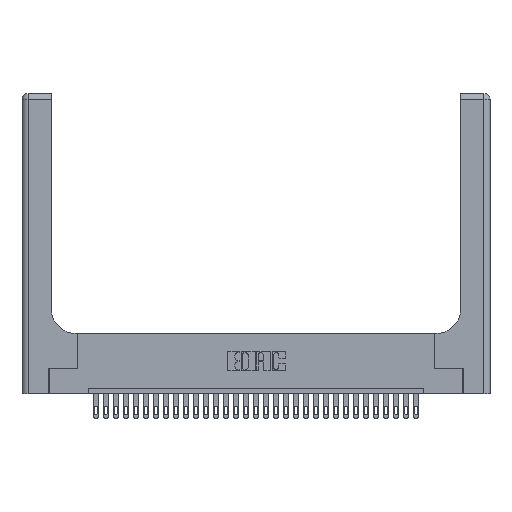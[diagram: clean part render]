
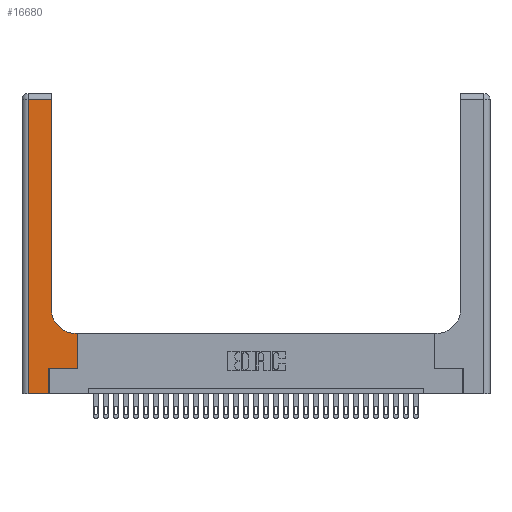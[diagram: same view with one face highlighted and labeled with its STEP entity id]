
A CAD part, top view. The second image highlights one B-rep face of the part: STEP entity #16680.
In plain terms, the highlighted planar face has unit normal (0, 0, 1).
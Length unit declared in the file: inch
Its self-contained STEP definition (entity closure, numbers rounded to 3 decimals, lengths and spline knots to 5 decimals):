
#653 = CARTESIAN_POINT ( 'NONE',  ( 0.2915, 3., 0.37 ) ) ;
#688 = VERTEX_POINT ( 'NONE', #6869 ) ;
#907 = DIRECTION ( 'NONE',  ( -1., 0., 0. ) ) ;
#1330 = ORIENTED_EDGE ( 'NONE', *, *, #17943, .T. ) ;
#1447 = CARTESIAN_POINT ( 'NONE',  ( 0.5415, 0.6, 0.37 ) ) ;
#1498 = DIRECTION ( 'NONE',  ( 0., 0., -1. ) ) ;
#3628 = CARTESIAN_POINT ( 'NONE',  ( 0.2915, 0.85, 0.37 ) ) ;
#3691 = LINE ( 'NONE', #653, #22106 ) ;
#4813 = PLANE ( 'NONE',  #30777 ) ;
#5582 = DIRECTION ( 'NONE',  ( 0., 1., 0. ) ) ;
#5802 = VECTOR ( 'NONE', #12513, 39.37008 ) ;
#6184 = VERTEX_POINT ( 'NONE', #26454 ) ;
#6189 = EDGE_CURVE ( 'NONE', #15887, #24402, #13624, .T. ) ;
#6240 = VECTOR ( 'NONE', #15672, 39.37008 ) ;
#6869 = CARTESIAN_POINT ( 'NONE',  ( 0.5585, 0.25, 0.37 ) ) ;
#6893 = CARTESIAN_POINT ( 'NONE',  ( 0., 0., 0.37 ) ) ;
#6897 = ORIENTED_EDGE ( 'NONE', *, *, #6189, .T. ) ;
#6902 = LINE ( 'NONE', #23848, #26499 ) ;
#6960 = DIRECTION ( 'NONE',  ( 1., 0., 0. ) ) ;
#7021 = AXIS2_PLACEMENT_3D ( 'NONE', #13616, #1498, #25425 ) ;
#7666 = DIRECTION ( 'NONE',  ( -1., 0., 0. ) ) ;
#7793 = VERTEX_POINT ( 'NONE', #1447 ) ;
#8768 = ORIENTED_EDGE ( 'NONE', *, *, #16784, .T. ) ;
#9126 = VECTOR ( 'NONE', #907, 39.37008 ) ;
#10651 = VECTOR ( 'NONE', #16989, 39.37008 ) ;
#10754 = EDGE_CURVE ( 'NONE', #24402, #30688, #6902, .T. ) ;
#11161 = EDGE_CURVE ( 'NONE', #7793, #23447, #12227, .T. ) ;
#11666 = LINE ( 'NONE', #14273, #12425 ) ;
#11920 = DIRECTION ( 'NONE',  ( 0., -1., 0. ) ) ;
#12227 = CIRCLE ( 'NONE', #7021, 0.25 ) ;
#12425 = VECTOR ( 'NONE', #6960, 39.37008 ) ;
#12513 = DIRECTION ( 'NONE',  ( 0., 1., 0. ) ) ;
#13601 = EDGE_LOOP ( 'NONE', ( #8768, #25723, #25449, #6897, #31144, #28677, #14193, #1330, #15732 ) ) ;
#13616 = CARTESIAN_POINT ( 'NONE',  ( 0.5415, 0.85, 0.37 ) ) ;
#13624 = LINE ( 'NONE', #6893, #10651 ) ;
#14193 = ORIENTED_EDGE ( 'NONE', *, *, #29906, .T. ) ;
#14273 = CARTESIAN_POINT ( 'NONE',  ( 0.269, 0.25, 0.37 ) ) ;
#14538 = EDGE_CURVE ( 'NONE', #21048, #15887, #25951, .T. ) ;
#15152 = CARTESIAN_POINT ( 'NONE',  ( 0.2915, 0.6, 0.37 ) ) ;
#15672 = DIRECTION ( 'NONE',  ( -1., 0., 0. ) ) ;
#15732 = ORIENTED_EDGE ( 'NONE', *, *, #11161, .T. ) ;
#15887 = VERTEX_POINT ( 'NONE', #17524 ) ;
#15949 = VERTEX_POINT ( 'NONE', #25364 ) ;
#16680 = ADVANCED_FACE ( 'NONE', ( #27053 ), #4813, .F. ) ;
#16784 = EDGE_CURVE ( 'NONE', #23447, #15949, #3691, .T. ) ;
#16989 = DIRECTION ( 'NONE',  ( 1., 0., 0. ) ) ;
#17524 = CARTESIAN_POINT ( 'NONE',  ( 0.06, 0., 0.37 ) ) ;
#17818 = LINE ( 'NONE', #24427, #5802 ) ;
#17943 = EDGE_CURVE ( 'NONE', #6184, #7793, #22686, .T. ) ;
#18243 = CARTESIAN_POINT ( 'NONE',  ( 0.269, 0.25, 0.37 ) ) ;
#19518 = EDGE_CURVE ( 'NONE', #30688, #688, #11666, .T. ) ;
#20526 = LINE ( 'NONE', #22747, #6240 ) ;
#21048 = VERTEX_POINT ( 'NONE', #30286 ) ;
#21851 = CARTESIAN_POINT ( 'NONE',  ( 0., 3., 0.37 ) ) ;
#22106 = VECTOR ( 'NONE', #5582, 39.37008 ) ;
#22244 = EDGE_CURVE ( 'NONE', #15949, #21048, #20526, .T. ) ;
#22686 = LINE ( 'NONE', #15152, #9126 ) ;
#22747 = CARTESIAN_POINT ( 'NONE',  ( 0., 2.94, 0.37 ) ) ;
#23447 = VERTEX_POINT ( 'NONE', #3628 ) ;
#23787 = DIRECTION ( 'NONE',  ( 0., 0., -1. ) ) ;
#23848 = CARTESIAN_POINT ( 'NONE',  ( 0.269, 0., 0.37 ) ) ;
#24402 = VERTEX_POINT ( 'NONE', #24681 ) ;
#24427 = CARTESIAN_POINT ( 'NONE',  ( 0.5585, 0.25, 0.37 ) ) ;
#24681 = CARTESIAN_POINT ( 'NONE',  ( 0.269, 0., 0.37 ) ) ;
#25364 = CARTESIAN_POINT ( 'NONE',  ( 0.2915, 2.94, 0.37 ) ) ;
#25425 = DIRECTION ( 'NONE',  ( 1., 0., 0. ) ) ;
#25449 = ORIENTED_EDGE ( 'NONE', *, *, #14538, .T. ) ;
#25723 = ORIENTED_EDGE ( 'NONE', *, *, #22244, .T. ) ;
#25951 = LINE ( 'NONE', #28609, #26745 ) ;
#26454 = CARTESIAN_POINT ( 'NONE',  ( 0.5585, 0.6, 0.37 ) ) ;
#26499 = VECTOR ( 'NONE', #28412, 39.37008 ) ;
#26745 = VECTOR ( 'NONE', #11920, 39.37008 ) ;
#27053 = FACE_OUTER_BOUND ( 'NONE', #13601, .T. ) ;
#28412 = DIRECTION ( 'NONE',  ( 0., 1., 0. ) ) ;
#28609 = CARTESIAN_POINT ( 'NONE',  ( 0.06, 3., 0.37 ) ) ;
#28677 = ORIENTED_EDGE ( 'NONE', *, *, #19518, .T. ) ;
#29906 = EDGE_CURVE ( 'NONE', #688, #6184, #17818, .T. ) ;
#30286 = CARTESIAN_POINT ( 'NONE',  ( 0.06, 2.94, 0.37 ) ) ;
#30688 = VERTEX_POINT ( 'NONE', #18243 ) ;
#30777 = AXIS2_PLACEMENT_3D ( 'NONE', #21851, #23787, #7666 ) ;
#31144 = ORIENTED_EDGE ( 'NONE', *, *, #10754, .T. ) ;
